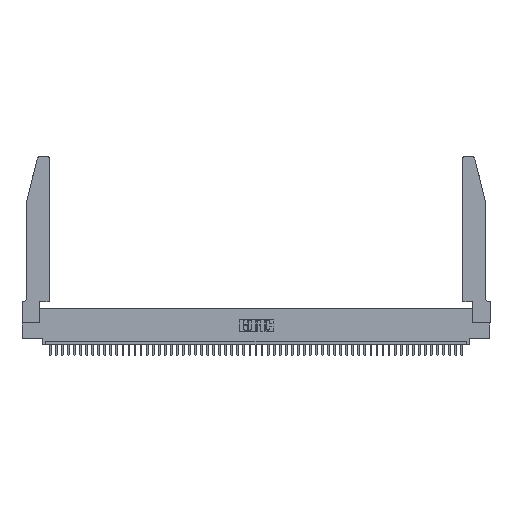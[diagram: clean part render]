
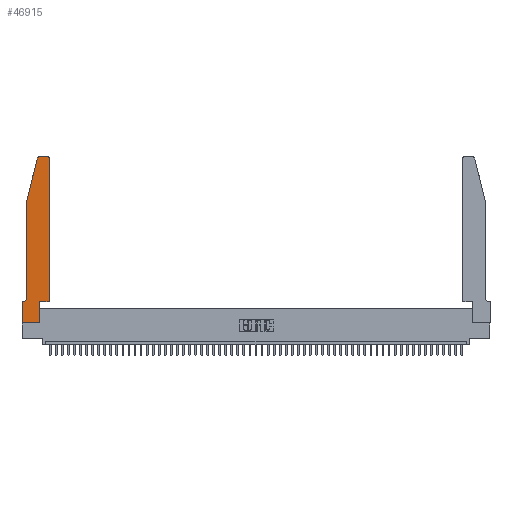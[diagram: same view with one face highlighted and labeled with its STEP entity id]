
A CAD part, top view. The second image highlights one B-rep face of the part: STEP entity #46915.
In plain terms, the highlighted planar face has unit normal (0, 0, 1).
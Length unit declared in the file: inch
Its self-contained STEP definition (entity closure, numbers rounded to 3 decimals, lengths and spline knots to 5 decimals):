
#552 = DIRECTION ( 'NONE',  ( -0.239, -0.971, 0. ) ) ;
#621 = EDGE_CURVE ( 'NONE', #44795, #44057, #51233, .T. ) ;
#1054 = VERTEX_POINT ( 'NONE', #21905 ) ;
#1888 = CARTESIAN_POINT ( 'NONE',  ( 0.4505, 0.35, 0.37 ) ) ;
#2291 = EDGE_CURVE ( 'NONE', #40295, #1054, #17608, .T. ) ;
#2371 = EDGE_CURVE ( 'NONE', #46289, #18675, #53101, .T. ) ;
#2519 = ORIENTED_EDGE ( 'NONE', *, *, #621, .T. ) ;
#3606 = ORIENTED_EDGE ( 'NONE', *, *, #36378, .T. ) ;
#3747 = VECTOR ( 'NONE', #36173, 39.37008 ) ;
#3753 = LINE ( 'NONE', #44172, #42981 ) ;
#4595 = CARTESIAN_POINT ( 'NONE',  ( 0.4505, 2.72, 0.37 ) ) ;
#5656 = ORIENTED_EDGE ( 'NONE', *, *, #2291, .T. ) ;
#5934 = CARTESIAN_POINT ( 'NONE',  ( 0.284, 2.75, 0.37 ) ) ;
#7846 = EDGE_CURVE ( 'NONE', #18675, #19837, #3753, .T. ) ;
#8421 = EDGE_CURVE ( 'NONE', #43628, #40295, #10161, .T. ) ;
#8425 = DIRECTION ( 'NONE',  ( 1., 0., 0. ) ) ;
#8625 = AXIS2_PLACEMENT_3D ( 'NONE', #11917, #24341, #20509 ) ;
#8826 = AXIS2_PLACEMENT_3D ( 'NONE', #32903, #37214, #8425 ) ;
#9437 = CARTESIAN_POINT ( 'NONE',  ( 0.0755, 2., 0.37 ) ) ;
#9495 = ORIENTED_EDGE ( 'NONE', *, *, #7846, .T. ) ;
#9819 = CARTESIAN_POINT ( 'NONE',  ( 0.4505, 0.35, 0.37 ) ) ;
#10161 = LINE ( 'NONE', #1888, #12785 ) ;
#10200 = LINE ( 'NONE', #42845, #24422 ) ;
#10235 = LINE ( 'NONE', #17135, #47624 ) ;
#10515 = CARTESIAN_POINT ( 'NONE',  ( 0.2865, 0.35, 0.37 ) ) ;
#11497 = DIRECTION ( 'NONE',  ( 0., -1., 0. ) ) ;
#11664 = FACE_OUTER_BOUND ( 'NONE', #30577, .T. ) ;
#11917 = CARTESIAN_POINT ( 'NONE',  ( 0.284, 2.72, 0.37 ) ) ;
#12785 = VECTOR ( 'NONE', #26978, 39.37008 ) ;
#14009 = LINE ( 'NONE', #10515, #3747 ) ;
#14842 = EDGE_CURVE ( 'NONE', #1054, #44795, #10200, .T. ) ;
#15203 = CARTESIAN_POINT ( 'NONE',  ( 0.0755, 0.35, 0.37 ) ) ;
#15574 = CARTESIAN_POINT ( 'NONE',  ( 0., 0., 0.37 ) ) ;
#17135 = CARTESIAN_POINT ( 'NONE',  ( 0.0755, 2., 0.37 ) ) ;
#17608 = CIRCLE ( 'NONE', #38611, 0.03 ) ;
#18675 = VERTEX_POINT ( 'NONE', #15574 ) ;
#18682 = ORIENTED_EDGE ( 'NONE', *, *, #46997, .T. ) ;
#18785 = VECTOR ( 'NONE', #52465, 39.37008 ) ;
#19837 = VERTEX_POINT ( 'NONE', #20928 ) ;
#20341 = VERTEX_POINT ( 'NONE', #28026 ) ;
#20509 = DIRECTION ( 'NONE',  ( 1., 0., 0. ) ) ;
#20928 = CARTESIAN_POINT ( 'NONE',  ( 0.2865, 0., 0.37 ) ) ;
#21905 = CARTESIAN_POINT ( 'NONE',  ( 0.4205, 2.75, 0.37 ) ) ;
#22304 = DIRECTION ( 'NONE',  ( -1., 0., 0. ) ) ;
#22962 = EDGE_CURVE ( 'NONE', #19837, #29594, #14009, .T. ) ;
#23377 = VECTOR ( 'NONE', #552, 39.37008 ) ;
#23738 = CARTESIAN_POINT ( 'NONE',  ( 0.0055, 0.42, 0.37 ) ) ;
#24341 = DIRECTION ( 'NONE',  ( 0., 0., 1. ) ) ;
#24413 = AXIS2_PLACEMENT_3D ( 'NONE', #23738, #52323, #33078 ) ;
#24422 = VECTOR ( 'NONE', #22304, 39.37008 ) ;
#24643 = PLANE ( 'NONE',  #8826 ) ;
#24690 = LINE ( 'NONE', #9437, #23377 ) ;
#25939 = CARTESIAN_POINT ( 'NONE',  ( 0.0755, 0.42, 0.37 ) ) ;
#26978 = DIRECTION ( 'NONE',  ( 0., 1., 0. ) ) ;
#27011 = ORIENTED_EDGE ( 'NONE', *, *, #42969, .T. ) ;
#28026 = CARTESIAN_POINT ( 'NONE',  ( 0.0055, 0.35, 0.37 ) ) ;
#29097 = ORIENTED_EDGE ( 'NONE', *, *, #34386, .T. ) ;
#29241 = CARTESIAN_POINT ( 'NONE',  ( 0.25487, 2.72718, 0.37 ) ) ;
#29594 = VERTEX_POINT ( 'NONE', #32549 ) ;
#30458 = LINE ( 'NONE', #15203, #50994 ) ;
#30577 = EDGE_LOOP ( 'NONE', ( #48413, #2519, #29097, #3606, #18682, #27011, #35327, #9495, #35867, #32289, #48855, #5656 ) ) ;
#31533 = DIRECTION ( 'NONE',  ( 1., 0., 0. ) ) ;
#32289 = ORIENTED_EDGE ( 'NONE', *, *, #34756, .T. ) ;
#32373 = DIRECTION ( 'NONE',  ( 0., 0., 1. ) ) ;
#32549 = CARTESIAN_POINT ( 'NONE',  ( 0.2865, 0.35, 0.37 ) ) ;
#32706 = CARTESIAN_POINT ( 'NONE',  ( 0.4205, 2.72, 0.37 ) ) ;
#32903 = CARTESIAN_POINT ( 'NONE',  ( 0., 0.35, 0.37 ) ) ;
#33078 = DIRECTION ( 'NONE',  ( -1., 0., 0. ) ) ;
#34386 = EDGE_CURVE ( 'NONE', #44057, #37708, #24690, .T. ) ;
#34756 = EDGE_CURVE ( 'NONE', #29594, #43628, #43234, .T. ) ;
#35126 = CARTESIAN_POINT ( 'NONE',  ( 0., 0.35, 0.37 ) ) ;
#35327 = ORIENTED_EDGE ( 'NONE', *, *, #2371, .T. ) ;
#35867 = ORIENTED_EDGE ( 'NONE', *, *, #22962, .T. ) ;
#35965 = CARTESIAN_POINT ( 'NONE',  ( 0.4505, 0.35, 0.37 ) ) ;
#36173 = DIRECTION ( 'NONE',  ( 0., 1., 0. ) ) ;
#36378 = EDGE_CURVE ( 'NONE', #37708, #36498, #10235, .T. ) ;
#36498 = VERTEX_POINT ( 'NONE', #25939 ) ;
#37214 = DIRECTION ( 'NONE',  ( 0., 0., 1. ) ) ;
#37708 = VERTEX_POINT ( 'NONE', #46037 ) ;
#38611 = AXIS2_PLACEMENT_3D ( 'NONE', #32706, #32373, #40958 ) ;
#39923 = CARTESIAN_POINT ( 'NONE',  ( 0., 0., 0.37 ) ) ;
#40295 = VERTEX_POINT ( 'NONE', #4595 ) ;
#40958 = DIRECTION ( 'NONE',  ( 1., 0., 0. ) ) ;
#42072 = VECTOR ( 'NONE', #11497, 39.37008 ) ;
#42117 = DIRECTION ( 'NONE',  ( 0., -1., 0. ) ) ;
#42845 = CARTESIAN_POINT ( 'NONE',  ( 0.2605, 2.75, 0.37 ) ) ;
#42969 = EDGE_CURVE ( 'NONE', #20341, #46289, #30458, .T. ) ;
#42981 = VECTOR ( 'NONE', #31533, 39.37008 ) ;
#43234 = LINE ( 'NONE', #35965, #18785 ) ;
#43628 = VERTEX_POINT ( 'NONE', #9819 ) ;
#43979 = DIRECTION ( 'NONE',  ( -1., 0., 0. ) ) ;
#44057 = VERTEX_POINT ( 'NONE', #29241 ) ;
#44172 = CARTESIAN_POINT ( 'NONE',  ( 0., 0., 0.37 ) ) ;
#44795 = VERTEX_POINT ( 'NONE', #5934 ) ;
#45199 = CIRCLE ( 'NONE', #24413, 0.07 ) ;
#46037 = CARTESIAN_POINT ( 'NONE',  ( 0.0755, 2., 0.37 ) ) ;
#46289 = VERTEX_POINT ( 'NONE', #35126 ) ;
#46915 = ADVANCED_FACE ( 'NONE', ( #11664 ), #24643, .T. ) ;
#46997 = EDGE_CURVE ( 'NONE', #36498, #20341, #45199, .T. ) ;
#47624 = VECTOR ( 'NONE', #42117, 39.37008 ) ;
#48413 = ORIENTED_EDGE ( 'NONE', *, *, #14842, .T. ) ;
#48855 = ORIENTED_EDGE ( 'NONE', *, *, #8421, .T. ) ;
#50994 = VECTOR ( 'NONE', #43979, 39.37008 ) ;
#51233 = CIRCLE ( 'NONE', #8625, 0.03 ) ;
#52323 = DIRECTION ( 'NONE',  ( 0., 0., -1. ) ) ;
#52465 = DIRECTION ( 'NONE',  ( 1., 0., 0. ) ) ;
#53101 = LINE ( 'NONE', #39923, #42072 ) ;
